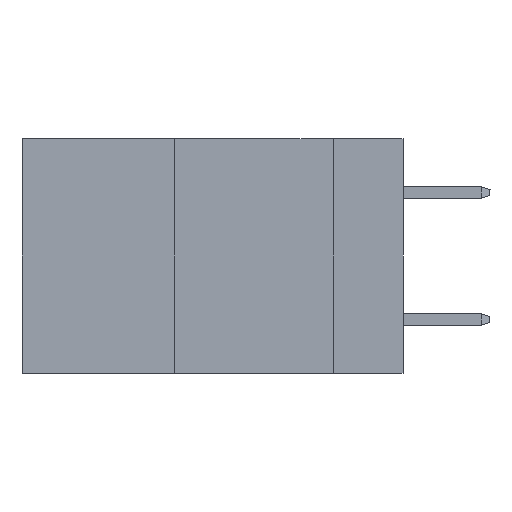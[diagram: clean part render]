
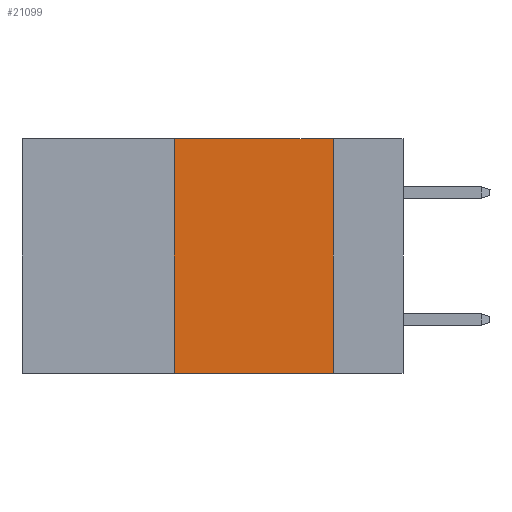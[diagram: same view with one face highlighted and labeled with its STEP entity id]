
A CAD part, left-side view. The second image highlights one B-rep face of the part: STEP entity #21099.
In plain terms, the highlighted planar face has unit normal (-1, 0, 0).
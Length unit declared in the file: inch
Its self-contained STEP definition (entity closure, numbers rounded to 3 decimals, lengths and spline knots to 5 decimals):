
#1536 = ORIENTED_EDGE ( 'NONE', *, *, #18230, .F. ) ;
#2364 = ORIENTED_EDGE ( 'NONE', *, *, #18276, .F. ) ;
#2820 = CARTESIAN_POINT ( 'NONE',  ( 0., 0.36, 0. ) ) ;
#4042 = VECTOR ( 'NONE', #17401, 39.37008 ) ;
#7721 = CARTESIAN_POINT ( 'NONE',  ( 0., 0.6, 0. ) ) ;
#8315 = EDGE_LOOP ( 'NONE', ( #2364, #1536, #26545, #23921 ) ) ;
#8900 = VERTEX_POINT ( 'NONE', #16660 ) ;
#12089 = PLANE ( 'NONE',  #14800 ) ;
#13537 = EDGE_CURVE ( 'NONE', #21539, #36517, #36527, .T. ) ;
#14800 = AXIS2_PLACEMENT_3D ( 'NONE', #25314, #22059, #25535 ) ;
#15311 = DIRECTION ( 'NONE',  ( 0., 0., -1. ) ) ;
#16660 = CARTESIAN_POINT ( 'NONE',  ( 0., 0.11, -0.37 ) ) ;
#17401 = DIRECTION ( 'NONE',  ( 0., 0., 1. ) ) ;
#18230 = EDGE_CURVE ( 'NONE', #36517, #36763, #37517, .T. ) ;
#18276 = EDGE_CURVE ( 'NONE', #36763, #8900, #31186, .T. ) ;
#20235 = CARTESIAN_POINT ( 'NONE',  ( 0., 0.11, 0. ) ) ;
#20285 = LINE ( 'NONE', #33083, #42506 ) ;
#20654 = CARTESIAN_POINT ( 'NONE',  ( 0., 0.36, 0. ) ) ;
#21099 = ADVANCED_FACE ( 'NONE', ( #35109 ), #12089, .F. ) ;
#21539 = VERTEX_POINT ( 'NONE', #36348 ) ;
#22059 = DIRECTION ( 'NONE',  ( 1., 0., 0. ) ) ;
#23921 = ORIENTED_EDGE ( 'NONE', *, *, #32802, .T. ) ;
#25314 = CARTESIAN_POINT ( 'NONE',  ( 0., 0.6, 0. ) ) ;
#25535 = DIRECTION ( 'NONE',  ( 0., 0., -1. ) ) ;
#26545 = ORIENTED_EDGE ( 'NONE', *, *, #13537, .F. ) ;
#31186 = LINE ( 'NONE', #41633, #32312 ) ;
#32312 = VECTOR ( 'NONE', #15311, 39.37008 ) ;
#32802 = EDGE_CURVE ( 'NONE', #21539, #8900, #20285, .T. ) ;
#33083 = CARTESIAN_POINT ( 'NONE',  ( 0., 0.6, -0.37 ) ) ;
#33590 = DIRECTION ( 'NONE',  ( 0., -1., 0. ) ) ;
#33727 = VECTOR ( 'NONE', #33590, 39.37008 ) ;
#35109 = FACE_OUTER_BOUND ( 'NONE', #8315, .T. ) ;
#36348 = CARTESIAN_POINT ( 'NONE',  ( 0., 0.36, -0.37 ) ) ;
#36517 = VERTEX_POINT ( 'NONE', #2820 ) ;
#36527 = LINE ( 'NONE', #20654, #4042 ) ;
#36763 = VERTEX_POINT ( 'NONE', #20235 ) ;
#37229 = DIRECTION ( 'NONE',  ( 0., -1., 0. ) ) ;
#37517 = LINE ( 'NONE', #7721, #33727 ) ;
#41633 = CARTESIAN_POINT ( 'NONE',  ( 0., 0.11, 0. ) ) ;
#42506 = VECTOR ( 'NONE', #37229, 39.37008 ) ;
